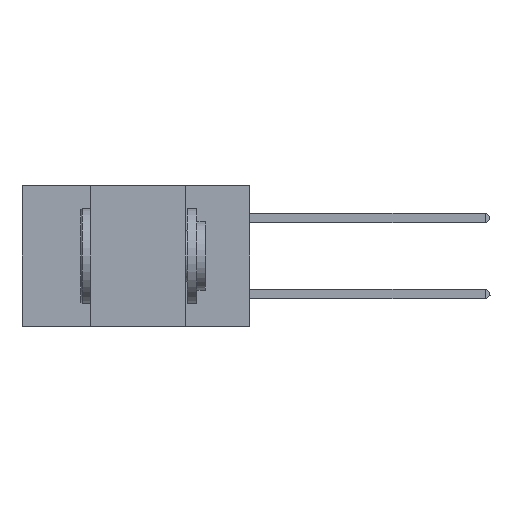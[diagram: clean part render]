
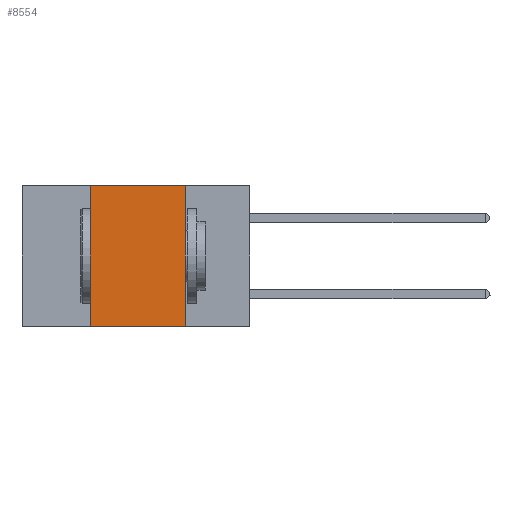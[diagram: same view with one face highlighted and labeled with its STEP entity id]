
A CAD part, left-side view. The second image highlights one B-rep face of the part: STEP entity #8554.
In plain terms, the highlighted planar face has unit normal (-1, 0, 0).
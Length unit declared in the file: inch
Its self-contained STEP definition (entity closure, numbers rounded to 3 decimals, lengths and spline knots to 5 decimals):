
#1100 = LINE ( 'NONE', #13624, #26040 ) ;
#1101 = EDGE_CURVE ( 'NONE', #4375, #17957, #20181, .T. ) ;
#2439 = ORIENTED_EDGE ( 'NONE', *, *, #19479, .F. ) ;
#2492 = CARTESIAN_POINT ( 'NONE',  ( 0., 0.17, 0. ) ) ;
#4023 = LINE ( 'NONE', #15436, #27321 ) ;
#4375 = VERTEX_POINT ( 'NONE', #12431 ) ;
#6304 = EDGE_CURVE ( 'NONE', #14850, #8804, #4023, .T. ) ;
#6387 = CARTESIAN_POINT ( 'NONE',  ( 0., 0.17, -0.37 ) ) ;
#6911 = CARTESIAN_POINT ( 'NONE',  ( 0., 0.42, 0. ) ) ;
#8053 = VECTOR ( 'NONE', #11287, 39.37008 ) ;
#8279 = ORIENTED_EDGE ( 'NONE', *, *, #8649, .T. ) ;
#8554 = ADVANCED_FACE ( 'NONE', ( #15068 ), #12578, .F. ) ;
#8606 = VECTOR ( 'NONE', #22943, 39.37008 ) ;
#8649 = EDGE_CURVE ( 'NONE', #4375, #8804, #25836, .T. ) ;
#8804 = VERTEX_POINT ( 'NONE', #6387 ) ;
#9535 = AXIS2_PLACEMENT_3D ( 'NONE', #21691, #24915, #21766 ) ;
#10824 = CARTESIAN_POINT ( 'NONE',  ( 0., 0.6, -0.37 ) ) ;
#11287 = DIRECTION ( 'NONE',  ( 0., 0., 1. ) ) ;
#12431 = CARTESIAN_POINT ( 'NONE',  ( 0., 0.42, -0.37 ) ) ;
#12565 = ORIENTED_EDGE ( 'NONE', *, *, #6304, .F. ) ;
#12578 = PLANE ( 'NONE',  #9535 ) ;
#13624 = CARTESIAN_POINT ( 'NONE',  ( 0., 0.6, 0. ) ) ;
#14850 = VERTEX_POINT ( 'NONE', #2492 ) ;
#15068 = FACE_OUTER_BOUND ( 'NONE', #17928, .T. ) ;
#15436 = CARTESIAN_POINT ( 'NONE',  ( 0., 0.17, 0. ) ) ;
#17384 = DIRECTION ( 'NONE',  ( 0., 0., -1. ) ) ;
#17928 = EDGE_LOOP ( 'NONE', ( #12565, #2439, #21618, #8279 ) ) ;
#17957 = VERTEX_POINT ( 'NONE', #18703 ) ;
#18703 = CARTESIAN_POINT ( 'NONE',  ( 0., 0.42, 0. ) ) ;
#19479 = EDGE_CURVE ( 'NONE', #17957, #14850, #1100, .T. ) ;
#20181 = LINE ( 'NONE', #6911, #8053 ) ;
#21618 = ORIENTED_EDGE ( 'NONE', *, *, #1101, .F. ) ;
#21691 = CARTESIAN_POINT ( 'NONE',  ( 0., 0.6, 0. ) ) ;
#21766 = DIRECTION ( 'NONE',  ( 0., 0., -1. ) ) ;
#22943 = DIRECTION ( 'NONE',  ( 0., -1., 0. ) ) ;
#24551 = DIRECTION ( 'NONE',  ( 0., -1., 0. ) ) ;
#24915 = DIRECTION ( 'NONE',  ( 1., 0., 0. ) ) ;
#25836 = LINE ( 'NONE', #10824, #8606 ) ;
#26040 = VECTOR ( 'NONE', #24551, 39.37008 ) ;
#27321 = VECTOR ( 'NONE', #17384, 39.37008 ) ;
